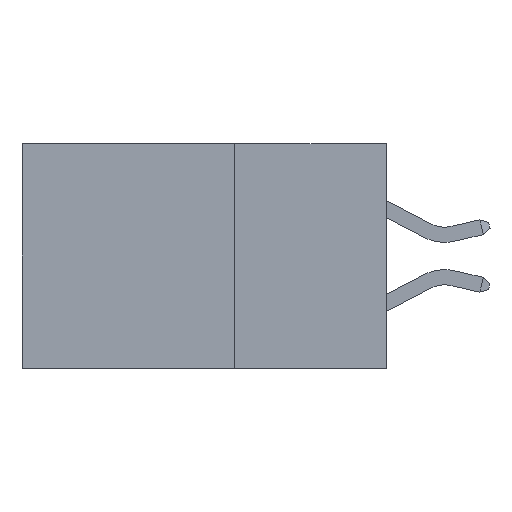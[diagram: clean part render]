
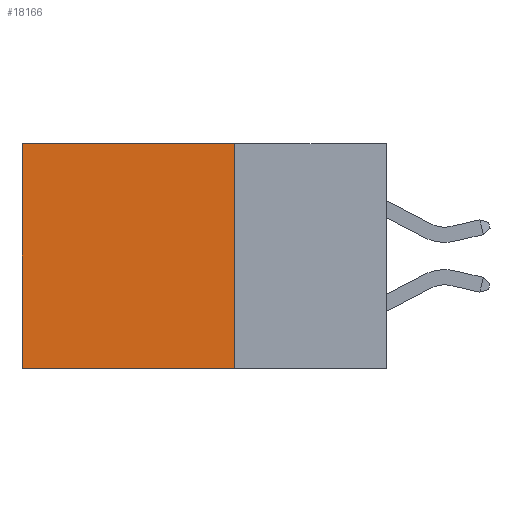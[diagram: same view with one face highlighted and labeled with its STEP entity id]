
A CAD part, left-side view. The second image highlights one B-rep face of the part: STEP entity #18166.
In plain terms, the highlighted planar face has unit normal (-1, 0, 0).
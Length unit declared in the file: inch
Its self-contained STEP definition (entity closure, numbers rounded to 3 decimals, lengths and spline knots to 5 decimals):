
#1883 = EDGE_CURVE ( 'NONE', #20335, #5239, #6150, .T. ) ;
#2282 = ORIENTED_EDGE ( 'NONE', *, *, #1883, .T. ) ;
#3260 = ORIENTED_EDGE ( 'NONE', *, *, #12596, .F. ) ;
#4186 = ORIENTED_EDGE ( 'NONE', *, *, #19241, .F. ) ;
#4404 = DIRECTION ( 'NONE',  ( 0., 0., -1. ) ) ;
#4460 = LINE ( 'NONE', #18335, #17720 ) ;
#4725 = VERTEX_POINT ( 'NONE', #8582 ) ;
#5239 = VERTEX_POINT ( 'NONE', #15899 ) ;
#5250 = EDGE_LOOP ( 'NONE', ( #21688, #3260, #4186, #2282 ) ) ;
#5770 = CARTESIAN_POINT ( 'NONE',  ( 0.298, 0.25, 0. ) ) ;
#6150 = LINE ( 'NONE', #5770, #10803 ) ;
#6347 = CARTESIAN_POINT ( 'NONE',  ( 0.298, 0.25, -0.37 ) ) ;
#6685 = VECTOR ( 'NONE', #13235, 39.37008 ) ;
#6933 = FACE_OUTER_BOUND ( 'NONE', #5250, .T. ) ;
#7257 = LINE ( 'NONE', #6347, #6685 ) ;
#8582 = CARTESIAN_POINT ( 'NONE',  ( 0.298, 0.25, -0.37 ) ) ;
#9031 = CARTESIAN_POINT ( 'NONE',  ( 0.298, 0.25, 0. ) ) ;
#9569 = CARTESIAN_POINT ( 'NONE',  ( 0.298, 0.6, 0. ) ) ;
#10239 = DIRECTION ( 'NONE',  ( 1., 0., 0. ) ) ;
#10803 = VECTOR ( 'NONE', #13977, 39.37008 ) ;
#11187 = CARTESIAN_POINT ( 'NONE',  ( 0.298, 0.6, -0.37 ) ) ;
#12596 = EDGE_CURVE ( 'NONE', #4725, #21827, #7257, .T. ) ;
#13235 = DIRECTION ( 'NONE',  ( 0., 1., 0. ) ) ;
#13826 = LINE ( 'NONE', #9569, #18371 ) ;
#13977 = DIRECTION ( 'NONE',  ( 0., 1., 0. ) ) ;
#15899 = CARTESIAN_POINT ( 'NONE',  ( 0.298, 0.6, 0. ) ) ;
#16052 = EDGE_CURVE ( 'NONE', #5239, #21827, #13826, .T. ) ;
#17720 = VECTOR ( 'NONE', #21817, 39.37008 ) ;
#18166 = ADVANCED_FACE ( 'NONE', ( #6933 ), #20446, .F. ) ;
#18335 = CARTESIAN_POINT ( 'NONE',  ( 0.298, 0.25, 0. ) ) ;
#18371 = VECTOR ( 'NONE', #4404, 39.37008 ) ;
#18401 = AXIS2_PLACEMENT_3D ( 'NONE', #20517, #10239, #22216 ) ;
#19241 = EDGE_CURVE ( 'NONE', #20335, #4725, #4460, .T. ) ;
#20335 = VERTEX_POINT ( 'NONE', #9031 ) ;
#20446 = PLANE ( 'NONE',  #18401 ) ;
#20517 = CARTESIAN_POINT ( 'NONE',  ( 0.298, 0.25, 0. ) ) ;
#21688 = ORIENTED_EDGE ( 'NONE', *, *, #16052, .T. ) ;
#21817 = DIRECTION ( 'NONE',  ( 0., 0., -1. ) ) ;
#21827 = VERTEX_POINT ( 'NONE', #11187 ) ;
#22216 = DIRECTION ( 'NONE',  ( 0., 0., -1. ) ) ;
